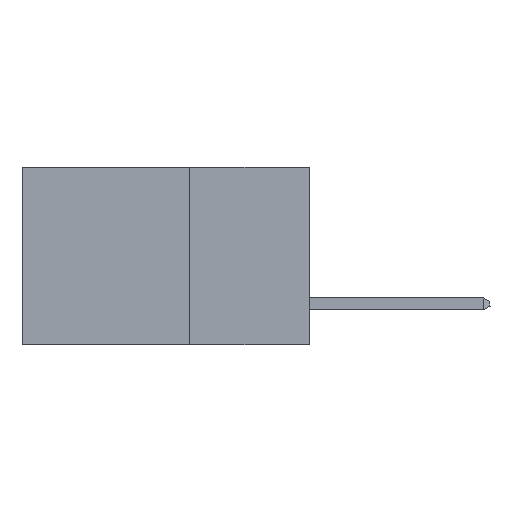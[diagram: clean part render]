
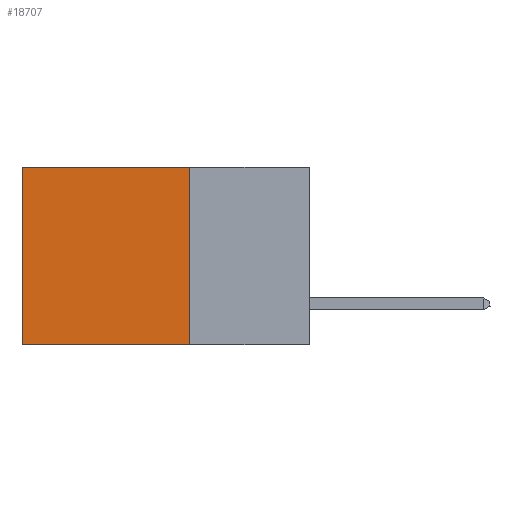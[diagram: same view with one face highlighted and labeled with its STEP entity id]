
A CAD part, left-side view. The second image highlights one B-rep face of the part: STEP entity #18707.
In plain terms, the highlighted planar face has unit normal (-1, 0, 0).
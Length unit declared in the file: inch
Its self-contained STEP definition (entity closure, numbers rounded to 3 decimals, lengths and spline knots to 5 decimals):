
#1244 = CARTESIAN_POINT ( 'NONE',  ( 0.2875, 0.25, 0. ) ) ;
#1326 = VECTOR ( 'NONE', #14446, 39.37008 ) ;
#1422 = CARTESIAN_POINT ( 'NONE',  ( 0.2875, 0.6, -0.37 ) ) ;
#1852 = CARTESIAN_POINT ( 'NONE',  ( 0.2875, 0.25, 0. ) ) ;
#2362 = VERTEX_POINT ( 'NONE', #1422 ) ;
#3851 = VECTOR ( 'NONE', #15319, 39.37008 ) ;
#4434 = VERTEX_POINT ( 'NONE', #16675 ) ;
#6249 = LINE ( 'NONE', #8772, #1326 ) ;
#7085 = CARTESIAN_POINT ( 'NONE',  ( 0.2875, 0.25, 0. ) ) ;
#7097 = AXIS2_PLACEMENT_3D ( 'NONE', #7085, #19920, #18288 ) ;
#7311 = ORIENTED_EDGE ( 'NONE', *, *, #20757, .T. ) ;
#7509 = CARTESIAN_POINT ( 'NONE',  ( 0.2875, 0.6, 0. ) ) ;
#8772 = CARTESIAN_POINT ( 'NONE',  ( 0.2875, 0.25, 0. ) ) ;
#8871 = EDGE_LOOP ( 'NONE', ( #7311, #21885, #16171, #16128 ) ) ;
#9254 = EDGE_CURVE ( 'NONE', #4434, #2362, #17784, .T. ) ;
#10128 = CARTESIAN_POINT ( 'NONE',  ( 0.2875, 0.6, 0. ) ) ;
#11140 = DIRECTION ( 'NONE',  ( 0., 0., -1. ) ) ;
#12130 = DIRECTION ( 'NONE',  ( 0., 1., 0. ) ) ;
#12531 = VECTOR ( 'NONE', #11140, 39.37008 ) ;
#12794 = VERTEX_POINT ( 'NONE', #10128 ) ;
#12797 = VECTOR ( 'NONE', #12130, 39.37008 ) ;
#12998 = VERTEX_POINT ( 'NONE', #1244 ) ;
#13394 = LINE ( 'NONE', #1852, #12531 ) ;
#14422 = PLANE ( 'NONE',  #7097 ) ;
#14446 = DIRECTION ( 'NONE',  ( 0., 1., 0. ) ) ;
#15319 = DIRECTION ( 'NONE',  ( 0., 0., -1. ) ) ;
#15815 = CARTESIAN_POINT ( 'NONE',  ( 0.2875, 0.25, -0.37 ) ) ;
#16128 = ORIENTED_EDGE ( 'NONE', *, *, #23930, .T. ) ;
#16171 = ORIENTED_EDGE ( 'NONE', *, *, #22155, .F. ) ;
#16675 = CARTESIAN_POINT ( 'NONE',  ( 0.2875, 0.25, -0.37 ) ) ;
#17784 = LINE ( 'NONE', #15815, #12797 ) ;
#18288 = DIRECTION ( 'NONE',  ( 0., 0., -1. ) ) ;
#18707 = ADVANCED_FACE ( 'NONE', ( #23859 ), #14422, .F. ) ;
#19920 = DIRECTION ( 'NONE',  ( 1., 0., 0. ) ) ;
#20757 = EDGE_CURVE ( 'NONE', #12794, #2362, #23428, .T. ) ;
#21885 = ORIENTED_EDGE ( 'NONE', *, *, #9254, .F. ) ;
#22155 = EDGE_CURVE ( 'NONE', #12998, #4434, #13394, .T. ) ;
#23428 = LINE ( 'NONE', #7509, #3851 ) ;
#23859 = FACE_OUTER_BOUND ( 'NONE', #8871, .T. ) ;
#23930 = EDGE_CURVE ( 'NONE', #12998, #12794, #6249, .T. ) ;
